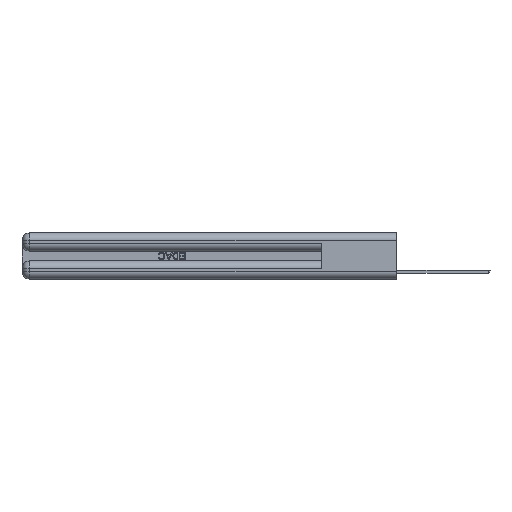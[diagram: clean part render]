
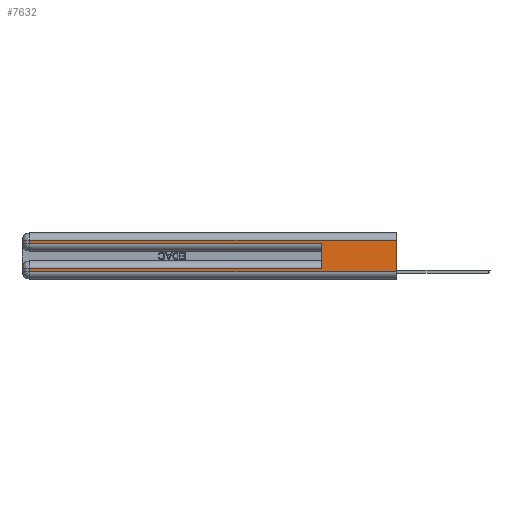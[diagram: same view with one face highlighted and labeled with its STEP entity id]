
A CAD part, left-side view. The second image highlights one B-rep face of the part: STEP entity #7632.
In plain terms, the highlighted planar face has unit normal (-1, 0, 0).
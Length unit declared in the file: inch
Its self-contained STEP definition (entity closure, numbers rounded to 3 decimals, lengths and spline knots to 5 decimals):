
#571 = ORIENTED_EDGE ( 'NONE', *, *, #27298, .T. ) ;
#1394 = VECTOR ( 'NONE', #11281, 39.37008 ) ;
#1925 = VERTEX_POINT ( 'NONE', #15677 ) ;
#2428 = ORIENTED_EDGE ( 'NONE', *, *, #9890, .F. ) ;
#3930 = CARTESIAN_POINT ( 'NONE',  ( 0., 0., 0.31 ) ) ;
#4166 = VECTOR ( 'NONE', #23380, 39.37008 ) ;
#4450 = VERTEX_POINT ( 'NONE', #20156 ) ;
#4970 = DIRECTION ( 'NONE',  ( 0., 0., -1. ) ) ;
#5168 = VECTOR ( 'NONE', #8403, 39.37008 ) ;
#5402 = CARTESIAN_POINT ( 'NONE',  ( 0., 0., 0.31 ) ) ;
#5700 = VECTOR ( 'NONE', #13590, 39.37008 ) ;
#6716 = CARTESIAN_POINT ( 'NONE',  ( 0., 0., 0.37 ) ) ;
#6755 = VERTEX_POINT ( 'NONE', #17172 ) ;
#6781 = VECTOR ( 'NONE', #19894, 39.37008 ) ;
#7632 = ADVANCED_FACE ( 'NONE', ( #31410 ), #29415, .F. ) ;
#8403 = DIRECTION ( 'NONE',  ( 0., 0., 1. ) ) ;
#8888 = VECTOR ( 'NONE', #25009, 39.37008 ) ;
#9369 = DIRECTION ( 'NONE',  ( 0., 0., -1. ) ) ;
#9890 = EDGE_CURVE ( 'NONE', #22075, #14600, #30835, .T. ) ;
#10263 = CARTESIAN_POINT ( 'NONE',  ( 0., 0., 0.06 ) ) ;
#10468 = CARTESIAN_POINT ( 'NONE',  ( 0., 0., 0.085 ) ) ;
#10761 = CARTESIAN_POINT ( 'NONE',  ( 0., 0., 0.285 ) ) ;
#11281 = DIRECTION ( 'NONE',  ( 0., -1., 0. ) ) ;
#11303 = EDGE_CURVE ( 'NONE', #12035, #4450, #29047, .T. ) ;
#12035 = VERTEX_POINT ( 'NONE', #19424 ) ;
#12320 = CARTESIAN_POINT ( 'NONE',  ( 0., 0., 0.06 ) ) ;
#12767 = DIRECTION ( 'NONE',  ( 0., 1., 0. ) ) ;
#12963 = EDGE_LOOP ( 'NONE', ( #2428, #14265, #13477, #30039, #32861, #25218, #24938, #571 ) ) ;
#13126 = DIRECTION ( 'NONE',  ( 1., 0., 0. ) ) ;
#13477 = ORIENTED_EDGE ( 'NONE', *, *, #34765, .T. ) ;
#13590 = DIRECTION ( 'NONE',  ( 0., 0., -1. ) ) ;
#13739 = LINE ( 'NONE', #32325, #5168 ) ;
#14265 = ORIENTED_EDGE ( 'NONE', *, *, #18607, .T. ) ;
#14439 = EDGE_CURVE ( 'NONE', #1925, #15976, #21389, .T. ) ;
#14600 = VERTEX_POINT ( 'NONE', #12320 ) ;
#15626 = VERTEX_POINT ( 'NONE', #31346 ) ;
#15677 = CARTESIAN_POINT ( 'NONE',  ( 0., 2.94, 0.285 ) ) ;
#15813 = CARTESIAN_POINT ( 'NONE',  ( 0., 0., 0.37 ) ) ;
#15976 = VERTEX_POINT ( 'NONE', #19843 ) ;
#16627 = EDGE_CURVE ( 'NONE', #12035, #15976, #13739, .T. ) ;
#17172 = CARTESIAN_POINT ( 'NONE',  ( 0., 2.94, 0.06 ) ) ;
#18607 = EDGE_CURVE ( 'NONE', #22075, #15626, #20256, .T. ) ;
#19424 = CARTESIAN_POINT ( 'NONE',  ( 0., 0.6, 0.085 ) ) ;
#19843 = CARTESIAN_POINT ( 'NONE',  ( 0., 0.6, 0.285 ) ) ;
#19894 = DIRECTION ( 'NONE',  ( 0., 1., 0. ) ) ;
#20156 = CARTESIAN_POINT ( 'NONE',  ( 0., 2.94, 0.085 ) ) ;
#20256 = LINE ( 'NONE', #3930, #6781 ) ;
#21389 = LINE ( 'NONE', #10761, #1394 ) ;
#21452 = VECTOR ( 'NONE', #12767, 39.37008 ) ;
#22075 = VERTEX_POINT ( 'NONE', #5402 ) ;
#23380 = DIRECTION ( 'NONE',  ( 0., -1., 0. ) ) ;
#24809 = LINE ( 'NONE', #27977, #26816 ) ;
#24938 = ORIENTED_EDGE ( 'NONE', *, *, #27769, .T. ) ;
#25009 = DIRECTION ( 'NONE',  ( 0., 0., -1. ) ) ;
#25218 = ORIENTED_EDGE ( 'NONE', *, *, #11303, .T. ) ;
#26816 = VECTOR ( 'NONE', #9369, 39.37008 ) ;
#26897 = LINE ( 'NONE', #27061, #5700 ) ;
#27061 = CARTESIAN_POINT ( 'NONE',  ( 0., 2.94, 0.37 ) ) ;
#27298 = EDGE_CURVE ( 'NONE', #6755, #14600, #34564, .T. ) ;
#27769 = EDGE_CURVE ( 'NONE', #4450, #6755, #26897, .T. ) ;
#27977 = CARTESIAN_POINT ( 'NONE',  ( 0., 2.94, 0.37 ) ) ;
#29047 = LINE ( 'NONE', #10468, #21452 ) ;
#29223 = AXIS2_PLACEMENT_3D ( 'NONE', #15813, #13126, #4970 ) ;
#29415 = PLANE ( 'NONE',  #29223 ) ;
#30039 = ORIENTED_EDGE ( 'NONE', *, *, #14439, .T. ) ;
#30835 = LINE ( 'NONE', #6716, #8888 ) ;
#31346 = CARTESIAN_POINT ( 'NONE',  ( 0., 2.94, 0.31 ) ) ;
#31410 = FACE_OUTER_BOUND ( 'NONE', #12963, .T. ) ;
#32325 = CARTESIAN_POINT ( 'NONE',  ( 0., 0.6, 0.145 ) ) ;
#32861 = ORIENTED_EDGE ( 'NONE', *, *, #16627, .F. ) ;
#34564 = LINE ( 'NONE', #10263, #4166 ) ;
#34765 = EDGE_CURVE ( 'NONE', #15626, #1925, #24809, .T. ) ;
